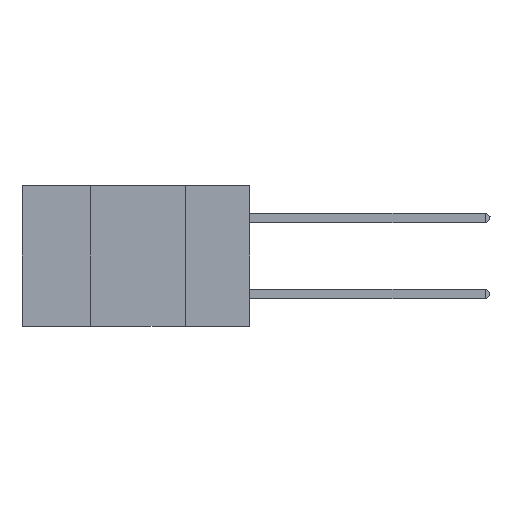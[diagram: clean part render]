
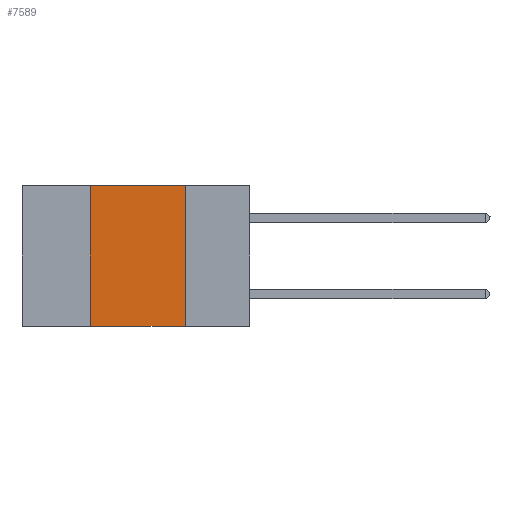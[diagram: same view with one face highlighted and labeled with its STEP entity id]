
A CAD part, left-side view. The second image highlights one B-rep face of the part: STEP entity #7589.
In plain terms, the highlighted planar face has unit normal (-1, 0, 0).
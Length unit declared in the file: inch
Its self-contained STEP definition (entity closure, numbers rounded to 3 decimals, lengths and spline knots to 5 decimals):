
#547 = VERTEX_POINT ( 'NONE', #7601 ) ;
#958 = ORIENTED_EDGE ( 'NONE', *, *, #10209, .T. ) ;
#1255 = VECTOR ( 'NONE', #9967, 39.37008 ) ;
#1338 = LINE ( 'NONE', #10684, #2436 ) ;
#1550 = VERTEX_POINT ( 'NONE', #7142 ) ;
#1612 = LINE ( 'NONE', #11168, #8275 ) ;
#2436 = VECTOR ( 'NONE', #2439, 39.37008 ) ;
#2439 = DIRECTION ( 'NONE',  ( 0., 0., 1. ) ) ;
#2470 = LINE ( 'NONE', #6250, #1255 ) ;
#2757 = DIRECTION ( 'NONE',  ( 0., 0., -1. ) ) ;
#3224 = EDGE_CURVE ( 'NONE', #1550, #7483, #1338, .T. ) ;
#3822 = CARTESIAN_POINT ( 'NONE',  ( 0., 0.17, -0.37 ) ) ;
#3899 = EDGE_CURVE ( 'NONE', #547, #3924, #5772, .T. ) ;
#3924 = VERTEX_POINT ( 'NONE', #3822 ) ;
#5501 = PLANE ( 'NONE',  #11930 ) ;
#5772 = LINE ( 'NONE', #10405, #5946 ) ;
#5946 = VECTOR ( 'NONE', #8628, 39.37008 ) ;
#6250 = CARTESIAN_POINT ( 'NONE',  ( 0., 0.6, -0.37 ) ) ;
#6268 = ORIENTED_EDGE ( 'NONE', *, *, #3899, .F. ) ;
#7142 = CARTESIAN_POINT ( 'NONE',  ( 0., 0.42, -0.37 ) ) ;
#7483 = VERTEX_POINT ( 'NONE', #9825 ) ;
#7589 = ADVANCED_FACE ( 'NONE', ( #11975 ), #5501, .F. ) ;
#7601 = CARTESIAN_POINT ( 'NONE',  ( 0., 0.17, 0. ) ) ;
#7948 = ORIENTED_EDGE ( 'NONE', *, *, #3224, .F. ) ;
#8275 = VECTOR ( 'NONE', #8361, 39.37008 ) ;
#8361 = DIRECTION ( 'NONE',  ( 0., -1., 0. ) ) ;
#8628 = DIRECTION ( 'NONE',  ( 0., 0., -1. ) ) ;
#9825 = CARTESIAN_POINT ( 'NONE',  ( 0., 0.42, 0. ) ) ;
#9909 = EDGE_LOOP ( 'NONE', ( #6268, #10589, #7948, #958 ) ) ;
#9967 = DIRECTION ( 'NONE',  ( 0., -1., 0. ) ) ;
#10008 = DIRECTION ( 'NONE',  ( 1., 0., 0. ) ) ;
#10094 = EDGE_CURVE ( 'NONE', #7483, #547, #1612, .T. ) ;
#10209 = EDGE_CURVE ( 'NONE', #1550, #3924, #2470, .T. ) ;
#10405 = CARTESIAN_POINT ( 'NONE',  ( 0., 0.17, 0. ) ) ;
#10589 = ORIENTED_EDGE ( 'NONE', *, *, #10094, .F. ) ;
#10684 = CARTESIAN_POINT ( 'NONE',  ( 0., 0.42, 0. ) ) ;
#11168 = CARTESIAN_POINT ( 'NONE',  ( 0., 0.6, 0. ) ) ;
#11916 = CARTESIAN_POINT ( 'NONE',  ( 0., 0.6, 0. ) ) ;
#11930 = AXIS2_PLACEMENT_3D ( 'NONE', #11916, #10008, #2757 ) ;
#11975 = FACE_OUTER_BOUND ( 'NONE', #9909, .T. ) ;
